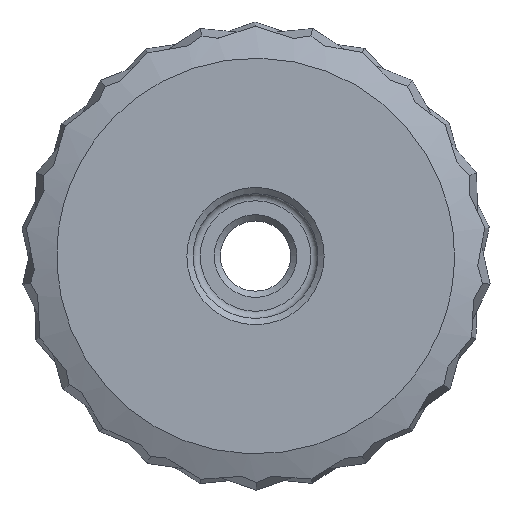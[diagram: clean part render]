
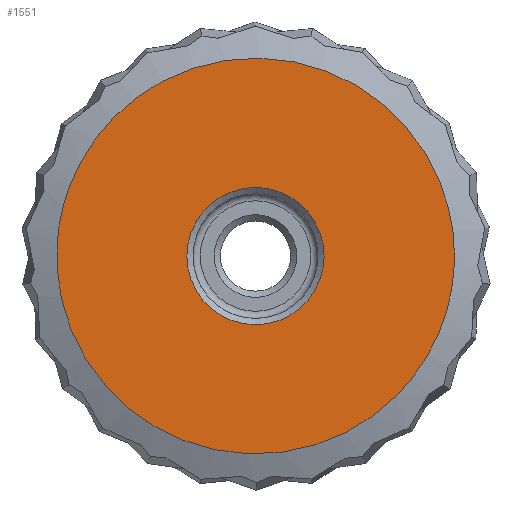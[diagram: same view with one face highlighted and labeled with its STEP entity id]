
A CAD part, front view. The second image highlights one B-rep face of the part: STEP entity #1551.
In plain terms, the highlighted planar face has unit normal (0, -1, 0).
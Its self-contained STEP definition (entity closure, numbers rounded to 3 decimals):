
#110 = DIRECTION ( 'NONE',  ( 1., 0., 0. ) ) ;
#378 = EDGE_CURVE ( 'NONE', #5195, #5195, #6003, .T. ) ;
#803 = DIRECTION ( 'NONE',  ( 0., 0., 1. ) ) ;
#1098 = AXIS2_PLACEMENT_3D ( 'NONE', #3190, #3112, #803 ) ;
#1206 = CARTESIAN_POINT ( 'NONE',  ( -391.941, 17.859, -0.281 ) ) ;
#1224 = ORIENTED_EDGE ( 'NONE', *, *, #378, .T. ) ;
#1256 = CARTESIAN_POINT ( 'NONE',  ( -404.679, 17.859, 25.087 ) ) ;
#1276 = CARTESIAN_POINT ( 'NONE',  ( -379.185, 17.859, -0.28 ) ) ;
#1432 = CARTESIAN_POINT ( 'NONE',  ( -379.185, 17.859, -0.28 ) ) ;
#1551 = ADVANCED_FACE ( 'NONE', ( #7297, #7098 ), #4370, .F. ) ;
#1827 = DIRECTION ( 'NONE',  ( 0., 1., 0. ) ) ;
#1848 = CARTESIAN_POINT ( 'NONE',  ( -379.185, 17.859, -0.28 ) ) ;
#1856 = EDGE_LOOP ( 'NONE', ( #1224 ) ) ;
#3110 = CARTESIAN_POINT ( 'NONE',  ( -404.679, 17.859, -25.647 ) ) ;
#3112 = DIRECTION ( 'NONE',  ( 0., 1., 0. ) ) ;
#3190 = CARTESIAN_POINT ( 'NONE',  ( -391.882, 17.859, -0.274 ) ) ;
#3510 = EDGE_LOOP ( 'NONE', ( #6869 ) ) ;
#3884 = EDGE_CURVE ( 'NONE', #6936, #6936, #4172, .T. ) ;
#4172 = CIRCLE ( 'NONE', #4466, 4.4 ) ;
#4370 = PLANE ( 'NONE',  #1098 ) ;
#4466 = AXIS2_PLACEMENT_3D ( 'NONE', #1206, #1827, #110 ) ;
#5195 = VERTEX_POINT ( 'NONE', #1432 ) ;
#5422 = CARTESIAN_POINT ( 'NONE',  ( -379.185, 17.859, 25.087 ) ) ;
#6003 =( BOUNDED_CURVE ( )  B_SPLINE_CURVE ( 3, ( #1848, #5422, #1256, #6628, #3110, #7180, #1276 ),
 .UNSPECIFIED., .T., .F. ) 
 B_SPLINE_CURVE_WITH_KNOTS ( ( 4, 3, 4 ),
 ( 0., 3.142, 6.283 ),
 .UNSPECIFIED. ) 
 CURVE ( )  GEOMETRIC_REPRESENTATION_ITEM ( )  RATIONAL_B_SPLINE_CURVE ( ( 1., 0.333, 0.333, 1., 0.333, 0.333, 1. ) ) 
 REPRESENTATION_ITEM ( '' )  );
#6628 = CARTESIAN_POINT ( 'NONE',  ( -404.679, 17.859, -0.28 ) ) ;
#6869 = ORIENTED_EDGE ( 'NONE', *, *, #3884, .T. ) ;
#6936 = VERTEX_POINT ( 'NONE', #7369 ) ;
#7098 = FACE_BOUND ( 'NONE', #3510, .T. ) ;
#7180 = CARTESIAN_POINT ( 'NONE',  ( -379.185, 17.859, -25.647 ) ) ;
#7297 = FACE_OUTER_BOUND ( 'NONE', #1856, .T. ) ;
#7369 = CARTESIAN_POINT ( 'NONE',  ( -387.541, 17.859, -0.281 ) ) ;
